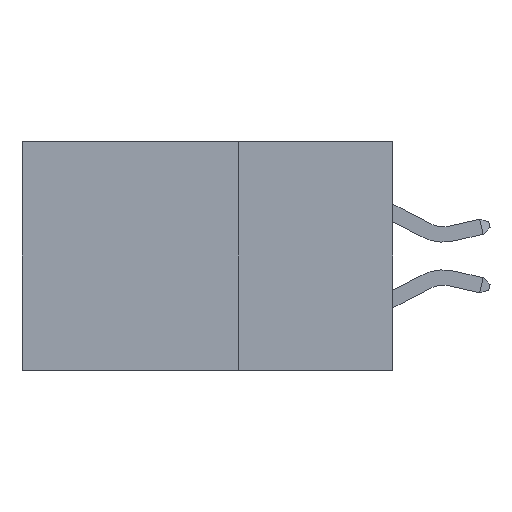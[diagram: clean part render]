
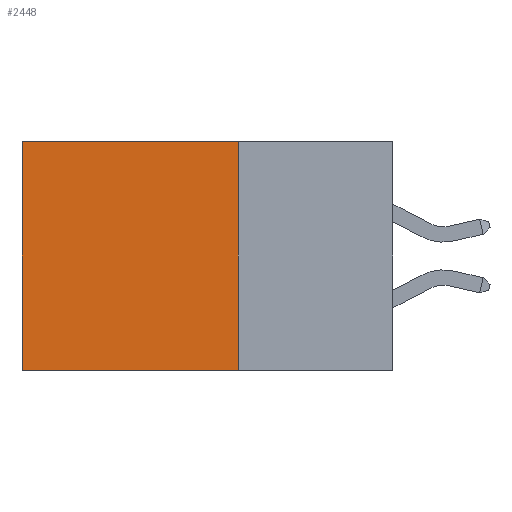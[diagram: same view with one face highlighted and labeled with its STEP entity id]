
A CAD part, left-side view. The second image highlights one B-rep face of the part: STEP entity #2448.
In plain terms, the highlighted planar face has unit normal (-1, 0, 0).
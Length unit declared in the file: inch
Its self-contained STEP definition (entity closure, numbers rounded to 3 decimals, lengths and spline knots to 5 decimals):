
#375 = FACE_OUTER_BOUND ( 'NONE', #10018, .T. ) ;
#399 = DIRECTION ( 'NONE',  ( 0., 0., -1. ) ) ;
#1090 = LINE ( 'NONE', #9461, #12483 ) ;
#1591 = PLANE ( 'NONE',  #9554 ) ;
#2448 = ADVANCED_FACE ( 'NONE', ( #375 ), #1591, .F. ) ;
#2553 = ORIENTED_EDGE ( 'NONE', *, *, #4343, .F. ) ;
#2588 = CARTESIAN_POINT ( 'NONE',  ( 0.2875, 0.25, 0. ) ) ;
#2625 = CARTESIAN_POINT ( 'NONE',  ( 0.2875, 0.6, 0. ) ) ;
#2695 = CARTESIAN_POINT ( 'NONE',  ( 0.2875, 0.25, -0.37 ) ) ;
#3058 = VERTEX_POINT ( 'NONE', #2625 ) ;
#4164 = EDGE_CURVE ( 'NONE', #3058, #7923, #1090, .T. ) ;
#4343 = EDGE_CURVE ( 'NONE', #7183, #7923, #7131, .T. ) ;
#4400 = DIRECTION ( 'NONE',  ( 0., 1., 0. ) ) ;
#4484 = CARTESIAN_POINT ( 'NONE',  ( 0.2875, 0.25, 0. ) ) ;
#4932 = ORIENTED_EDGE ( 'NONE', *, *, #5149, .F. ) ;
#5149 = EDGE_CURVE ( 'NONE', #7115, #7183, #10876, .T. ) ;
#5256 = VECTOR ( 'NONE', #12421, 39.37008 ) ;
#6522 = EDGE_CURVE ( 'NONE', #7115, #3058, #11786, .T. ) ;
#6926 = DIRECTION ( 'NONE',  ( 0., 1., 0. ) ) ;
#7115 = VERTEX_POINT ( 'NONE', #12677 ) ;
#7131 = LINE ( 'NONE', #11968, #9470 ) ;
#7183 = VERTEX_POINT ( 'NONE', #2695 ) ;
#7566 = DIRECTION ( 'NONE',  ( 0., 0., -1. ) ) ;
#7923 = VERTEX_POINT ( 'NONE', #7966 ) ;
#7966 = CARTESIAN_POINT ( 'NONE',  ( 0.2875, 0.6, -0.37 ) ) ;
#9461 = CARTESIAN_POINT ( 'NONE',  ( 0.2875, 0.6, 0. ) ) ;
#9470 = VECTOR ( 'NONE', #6926, 39.37008 ) ;
#9518 = DIRECTION ( 'NONE',  ( 1., 0., 0. ) ) ;
#9554 = AXIS2_PLACEMENT_3D ( 'NONE', #2588, #9518, #7566 ) ;
#10018 = EDGE_LOOP ( 'NONE', ( #12624, #2553, #4932, #12688 ) ) ;
#10876 = LINE ( 'NONE', #4484, #5256 ) ;
#11218 = CARTESIAN_POINT ( 'NONE',  ( 0.2875, 0.25, 0. ) ) ;
#11635 = VECTOR ( 'NONE', #4400, 39.37008 ) ;
#11786 = LINE ( 'NONE', #11218, #11635 ) ;
#11968 = CARTESIAN_POINT ( 'NONE',  ( 0.2875, 0.25, -0.37 ) ) ;
#12421 = DIRECTION ( 'NONE',  ( 0., 0., -1. ) ) ;
#12483 = VECTOR ( 'NONE', #399, 39.37008 ) ;
#12624 = ORIENTED_EDGE ( 'NONE', *, *, #4164, .T. ) ;
#12677 = CARTESIAN_POINT ( 'NONE',  ( 0.2875, 0.25, 0. ) ) ;
#12688 = ORIENTED_EDGE ( 'NONE', *, *, #6522, .T. ) ;
